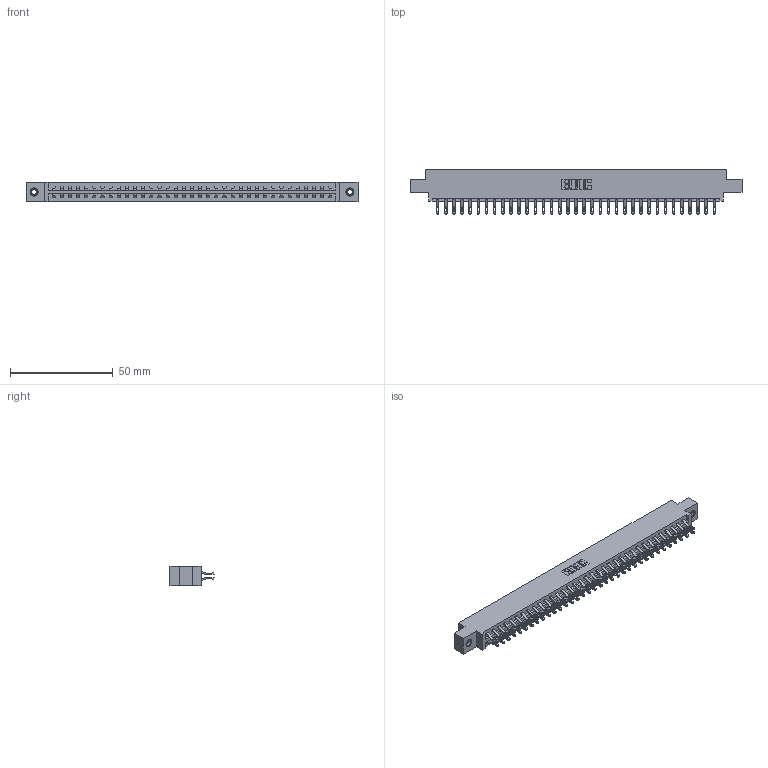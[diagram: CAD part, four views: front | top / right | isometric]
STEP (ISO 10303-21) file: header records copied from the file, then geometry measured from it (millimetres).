
FILE_DESCRIPTION (( 'STEP AP203' ), '1' );
FILE_NAME ('387-070-555-807.STEP', '2019-10-21T22:53:20', ( '' ), ( '' ), 'SwSTEP 2.0', 'SolidWorks 2016', '' );
FILE_SCHEMA (( 'CONFIG_CONTROL_DESIGN' ));
Length unit declared in the file: inch
Products named in the file (4): 387-070-555-807; 345-292-001_555 Tail; 345-250-001_345-250-005-103; 337 Part_0.170 Offset - 0.156 Dia-TI
Assembly tree (73 placements, depth 2):
  387-070-555-807
    337 Part_0.170 Offset - 0.156 Dia-TI
    345-292-001_555 Tail  x70
    345-250-001_345-250-005-103  x2
Bounding box: 161.7 x 21.47 x 9.4 mm (x, y, z)
Volume: 17019.7 mm3; surface area: 20081.7 mm2
Topology: 73 solids, 73 shells, 4378 faces, 13689 edges, 9118 vertices
Faces by surface type: plane 2626, cylinder 1736, cone 12, torus 4
Entity records: 29686 total; most frequent: CARTESIAN_POINT 5023, ORIENTED_EDGE 4922, DIRECTION 4287, EDGE_CURVE 2461, LINE 2293, VECTOR 2293, VERTEX_POINT 1636, AXIS2_PLACEMENT_3D 997
